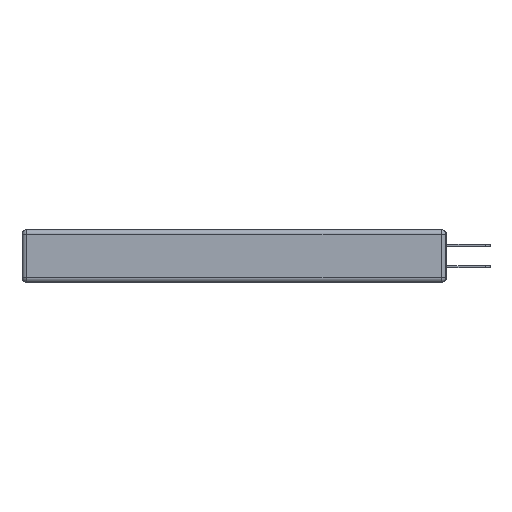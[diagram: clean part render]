
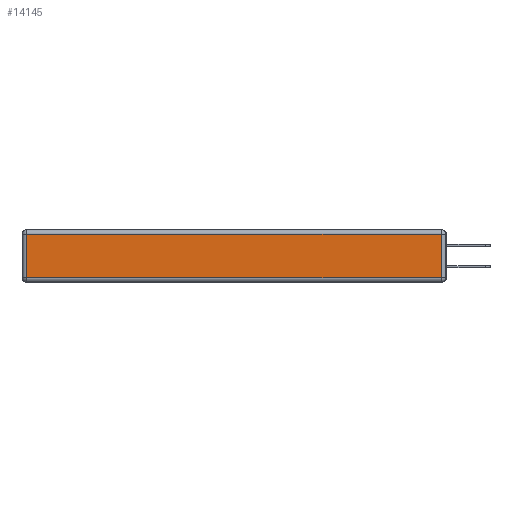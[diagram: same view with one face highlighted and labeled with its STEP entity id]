
A CAD part, left-side view. The second image highlights one B-rep face of the part: STEP entity #14145.
In plain terms, the highlighted planar face has unit normal (-1, 0, 0).
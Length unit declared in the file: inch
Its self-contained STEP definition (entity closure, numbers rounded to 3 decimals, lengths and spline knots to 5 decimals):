
#1194 = CARTESIAN_POINT ( 'NONE',  ( 0., 2.72, -0.313 ) ) ;
#1658 = VERTEX_POINT ( 'NONE', #1194 ) ;
#2768 = EDGE_CURVE ( 'NONE', #4055, #1658, #18583, .T. ) ;
#3734 = DIRECTION ( 'NONE',  ( 0., 0., -1. ) ) ;
#3845 = ORIENTED_EDGE ( 'NONE', *, *, #6665, .T. ) ;
#4055 = VERTEX_POINT ( 'NONE', #17256 ) ;
#4313 = CARTESIAN_POINT ( 'NONE',  ( 0., 0.03, -0.343 ) ) ;
#4865 = LINE ( 'NONE', #21008, #17446 ) ;
#6233 = EDGE_CURVE ( 'NONE', #22117, #15401, #13399, .T. ) ;
#6665 = EDGE_CURVE ( 'NONE', #15401, #4055, #7716, .T. ) ;
#7316 = DIRECTION ( 'NONE',  ( 0., 0., 1. ) ) ;
#7379 = DIRECTION ( 'NONE',  ( 0., 1., 0. ) ) ;
#7704 = CARTESIAN_POINT ( 'NONE',  ( 0., 2.72, -0.343 ) ) ;
#7716 = LINE ( 'NONE', #19332, #25361 ) ;
#7844 = AXIS2_PLACEMENT_3D ( 'NONE', #11729, #11454, #7316 ) ;
#7847 = EDGE_CURVE ( 'NONE', #1658, #22117, #4865, .T. ) ;
#9507 = ORIENTED_EDGE ( 'NONE', *, *, #6233, .T. ) ;
#11454 = DIRECTION ( 'NONE',  ( -1., 0., 0. ) ) ;
#11729 = CARTESIAN_POINT ( 'NONE',  ( 0., 0., -0.343 ) ) ;
#11851 = VECTOR ( 'NONE', #14259, 39.37008 ) ;
#13399 = LINE ( 'NONE', #4313, #11851 ) ;
#14145 = ADVANCED_FACE ( 'NONE', ( #22132 ), #25458, .T. ) ;
#14259 = DIRECTION ( 'NONE',  ( 0., 0., 1. ) ) ;
#15401 = VERTEX_POINT ( 'NONE', #16179 ) ;
#15492 = CARTESIAN_POINT ( 'NONE',  ( 0., 0.03, -0.313 ) ) ;
#16179 = CARTESIAN_POINT ( 'NONE',  ( 0., 0.03, -0.03 ) ) ;
#16377 = EDGE_LOOP ( 'NONE', ( #20188, #9507, #3845, #25768 ) ) ;
#17256 = CARTESIAN_POINT ( 'NONE',  ( 0., 2.72, -0.03 ) ) ;
#17446 = VECTOR ( 'NONE', #20852, 39.37008 ) ;
#18583 = LINE ( 'NONE', #7704, #19829 ) ;
#19332 = CARTESIAN_POINT ( 'NONE',  ( 0., 2.75, -0.03 ) ) ;
#19829 = VECTOR ( 'NONE', #3734, 39.37008 ) ;
#20188 = ORIENTED_EDGE ( 'NONE', *, *, #7847, .T. ) ;
#20852 = DIRECTION ( 'NONE',  ( 0., -1., 0. ) ) ;
#21008 = CARTESIAN_POINT ( 'NONE',  ( 0., 0., -0.313 ) ) ;
#22117 = VERTEX_POINT ( 'NONE', #15492 ) ;
#22132 = FACE_OUTER_BOUND ( 'NONE', #16377, .T. ) ;
#25361 = VECTOR ( 'NONE', #7379, 39.37008 ) ;
#25458 = PLANE ( 'NONE',  #7844 ) ;
#25768 = ORIENTED_EDGE ( 'NONE', *, *, #2768, .T. ) ;
